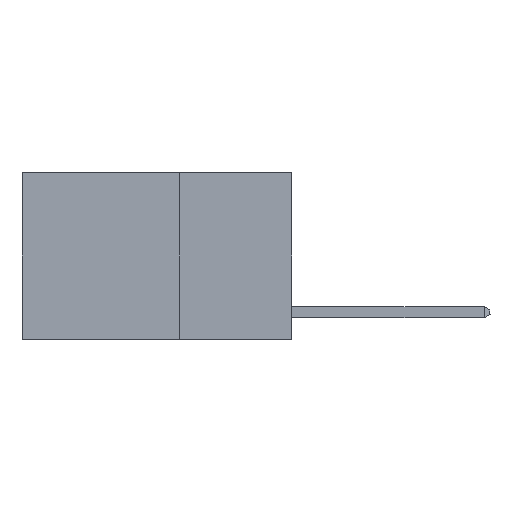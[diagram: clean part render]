
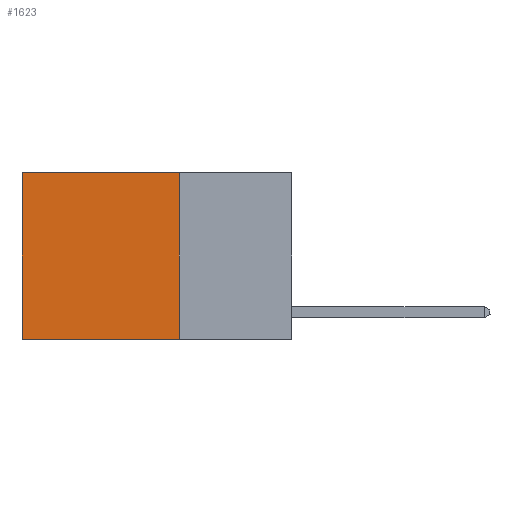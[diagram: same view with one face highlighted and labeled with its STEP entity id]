
A CAD part, left-side view. The second image highlights one B-rep face of the part: STEP entity #1623.
In plain terms, the highlighted planar face has unit normal (-1, 0, 0).
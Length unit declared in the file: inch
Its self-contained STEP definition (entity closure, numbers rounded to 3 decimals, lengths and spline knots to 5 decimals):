
#107 = LINE ( 'NONE', #3326, #666 ) ;
#268 = VECTOR ( 'NONE', #2733, 39.37008 ) ;
#517 = CARTESIAN_POINT ( 'NONE',  ( 0.2625, 0.25, 0. ) ) ;
#666 = VECTOR ( 'NONE', #1729, 39.37008 ) ;
#681 = VERTEX_POINT ( 'NONE', #3624 ) ;
#1265 = DIRECTION ( 'NONE',  ( 0., 0., -1. ) ) ;
#1286 = FACE_OUTER_BOUND ( 'NONE', #3545, .T. ) ;
#1468 = EDGE_CURVE ( 'NONE', #681, #6980, #4991, .T. ) ;
#1623 = ADVANCED_FACE ( 'NONE', ( #1286 ), #3800, .F. ) ;
#1651 = VERTEX_POINT ( 'NONE', #517 ) ;
#1729 = DIRECTION ( 'NONE',  ( 0., 1., 0. ) ) ;
#1993 = CARTESIAN_POINT ( 'NONE',  ( 0.2625, 0.25, 0. ) ) ;
#2032 = ORIENTED_EDGE ( 'NONE', *, *, #2382, .T. ) ;
#2105 = VECTOR ( 'NONE', #2640, 39.37008 ) ;
#2382 = EDGE_CURVE ( 'NONE', #1651, #681, #3505, .T. ) ;
#2640 = DIRECTION ( 'NONE',  ( 0., 1., 0. ) ) ;
#2724 = EDGE_CURVE ( 'NONE', #7916, #6980, #107, .T. ) ;
#2733 = DIRECTION ( 'NONE',  ( 0., 0., -1. ) ) ;
#3095 = VECTOR ( 'NONE', #1265, 39.37008 ) ;
#3326 = CARTESIAN_POINT ( 'NONE',  ( 0.2625, 0.25, -0.37 ) ) ;
#3505 = LINE ( 'NONE', #1993, #2105 ) ;
#3545 = EDGE_LOOP ( 'NONE', ( #6436, #5412, #9652, #2032 ) ) ;
#3624 = CARTESIAN_POINT ( 'NONE',  ( 0.2625, 0.6, 0. ) ) ;
#3800 = PLANE ( 'NONE',  #9918 ) ;
#4316 = LINE ( 'NONE', #9944, #3095 ) ;
#4991 = LINE ( 'NONE', #9155, #268 ) ;
#5360 = DIRECTION ( 'NONE',  ( 1., 0., 0. ) ) ;
#5412 = ORIENTED_EDGE ( 'NONE', *, *, #2724, .F. ) ;
#6095 = CARTESIAN_POINT ( 'NONE',  ( 0.2625, 0.25, 0. ) ) ;
#6436 = ORIENTED_EDGE ( 'NONE', *, *, #1468, .T. ) ;
#6754 = CARTESIAN_POINT ( 'NONE',  ( 0.2625, 0.6, -0.37 ) ) ;
#6944 = DIRECTION ( 'NONE',  ( 0., 0., -1. ) ) ;
#6980 = VERTEX_POINT ( 'NONE', #6754 ) ;
#7916 = VERTEX_POINT ( 'NONE', #10264 ) ;
#9155 = CARTESIAN_POINT ( 'NONE',  ( 0.2625, 0.6, 0. ) ) ;
#9410 = EDGE_CURVE ( 'NONE', #1651, #7916, #4316, .T. ) ;
#9652 = ORIENTED_EDGE ( 'NONE', *, *, #9410, .F. ) ;
#9918 = AXIS2_PLACEMENT_3D ( 'NONE', #6095, #5360, #6944 ) ;
#9944 = CARTESIAN_POINT ( 'NONE',  ( 0.2625, 0.25, 0. ) ) ;
#10264 = CARTESIAN_POINT ( 'NONE',  ( 0.2625, 0.25, -0.37 ) ) ;
